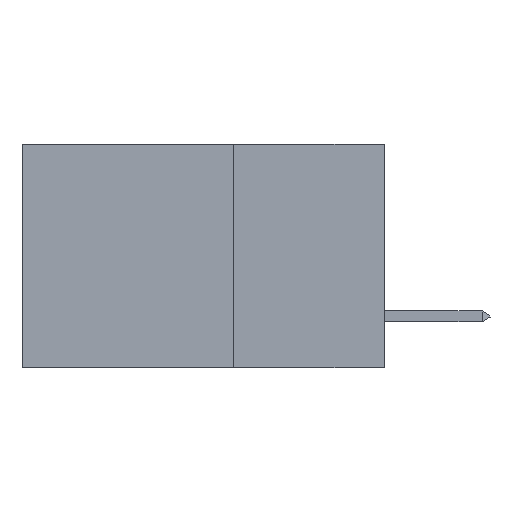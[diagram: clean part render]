
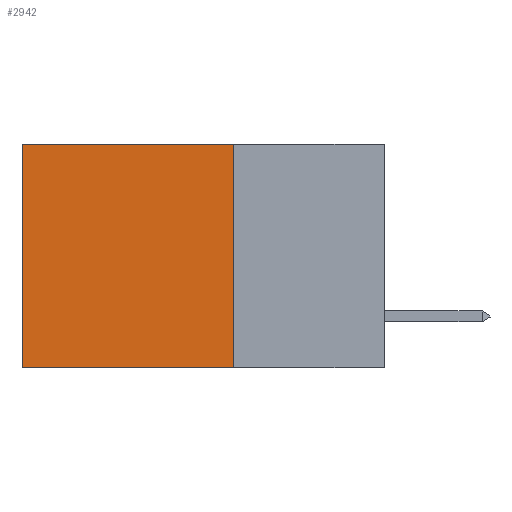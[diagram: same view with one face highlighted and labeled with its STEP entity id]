
A CAD part, left-side view. The second image highlights one B-rep face of the part: STEP entity #2942.
In plain terms, the highlighted planar face has unit normal (-1, 0, 0).
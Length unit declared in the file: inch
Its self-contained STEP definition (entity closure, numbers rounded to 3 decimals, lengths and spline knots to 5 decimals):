
#142 = EDGE_CURVE ( 'NONE', #6003, #1027, #1117, .T. ) ;
#230 = CARTESIAN_POINT ( 'NONE',  ( 0.2875, 0.25, 0. ) ) ;
#1027 = VERTEX_POINT ( 'NONE', #7653 ) ;
#1117 = LINE ( 'NONE', #1183, #11113 ) ;
#1183 = CARTESIAN_POINT ( 'NONE',  ( 0.2875, 0.25, 0. ) ) ;
#1436 = VECTOR ( 'NONE', #10775, 39.37008 ) ;
#2428 = CARTESIAN_POINT ( 'NONE',  ( 0.2875, 0.25, -0.37 ) ) ;
#2717 = FACE_OUTER_BOUND ( 'NONE', #10888, .T. ) ;
#2834 = ORIENTED_EDGE ( 'NONE', *, *, #5757, .F. ) ;
#2860 = LINE ( 'NONE', #6391, #10321 ) ;
#2942 = ADVANCED_FACE ( 'NONE', ( #2717 ), #7818, .F. ) ;
#3278 = DIRECTION ( 'NONE',  ( 0., 1., 0. ) ) ;
#5314 = VERTEX_POINT ( 'NONE', #11171 ) ;
#5757 = EDGE_CURVE ( 'NONE', #6003, #9413, #10982, .T. ) ;
#5986 = VECTOR ( 'NONE', #3278, 39.37008 ) ;
#6003 = VERTEX_POINT ( 'NONE', #7219 ) ;
#6261 = EDGE_CURVE ( 'NONE', #9413, #5314, #9794, .T. ) ;
#6391 = CARTESIAN_POINT ( 'NONE',  ( 0.2875, 0.6, 0. ) ) ;
#7109 = DIRECTION ( 'NONE',  ( 0., 1., 0. ) ) ;
#7219 = CARTESIAN_POINT ( 'NONE',  ( 0.2875, 0.25, 0. ) ) ;
#7377 = AXIS2_PLACEMENT_3D ( 'NONE', #10728, #12471, #9667 ) ;
#7653 = CARTESIAN_POINT ( 'NONE',  ( 0.2875, 0.6, 0. ) ) ;
#7818 = PLANE ( 'NONE',  #7377 ) ;
#7886 = ORIENTED_EDGE ( 'NONE', *, *, #142, .T. ) ;
#8369 = DIRECTION ( 'NONE',  ( 0., 0., -1. ) ) ;
#8979 = EDGE_CURVE ( 'NONE', #1027, #5314, #2860, .T. ) ;
#9413 = VERTEX_POINT ( 'NONE', #2428 ) ;
#9667 = DIRECTION ( 'NONE',  ( 0., 0., -1. ) ) ;
#9794 = LINE ( 'NONE', #9956, #5986 ) ;
#9889 = ORIENTED_EDGE ( 'NONE', *, *, #6261, .F. ) ;
#9956 = CARTESIAN_POINT ( 'NONE',  ( 0.2875, 0.25, -0.37 ) ) ;
#10321 = VECTOR ( 'NONE', #8369, 39.37008 ) ;
#10728 = CARTESIAN_POINT ( 'NONE',  ( 0.2875, 0.25, 0. ) ) ;
#10775 = DIRECTION ( 'NONE',  ( 0., 0., -1. ) ) ;
#10888 = EDGE_LOOP ( 'NONE', ( #11326, #9889, #2834, #7886 ) ) ;
#10982 = LINE ( 'NONE', #230, #1436 ) ;
#11113 = VECTOR ( 'NONE', #7109, 39.37008 ) ;
#11171 = CARTESIAN_POINT ( 'NONE',  ( 0.2875, 0.6, -0.37 ) ) ;
#11326 = ORIENTED_EDGE ( 'NONE', *, *, #8979, .T. ) ;
#12471 = DIRECTION ( 'NONE',  ( 1., 0., 0. ) ) ;
